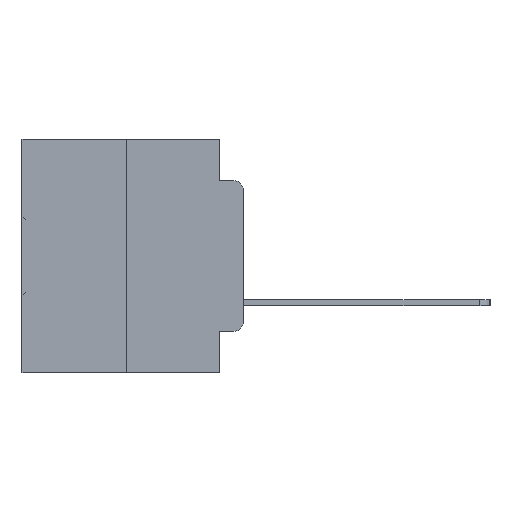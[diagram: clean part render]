
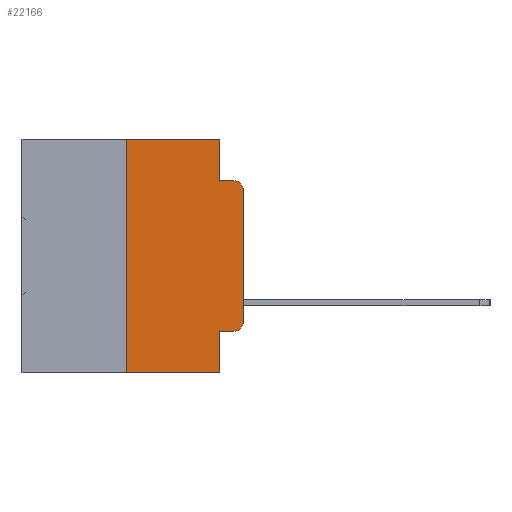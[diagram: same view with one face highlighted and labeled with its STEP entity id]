
A CAD part, left-side view. The second image highlights one B-rep face of the part: STEP entity #22166.
In plain terms, the highlighted planar face has unit normal (-1, 0, 0).
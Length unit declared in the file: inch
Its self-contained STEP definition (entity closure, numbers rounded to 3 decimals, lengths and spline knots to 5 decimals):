
#109 = DIRECTION ( 'NONE',  ( 0., 0., 1. ) ) ;
#383 = CARTESIAN_POINT ( 'NONE',  ( 0., 0.473, -0.5 ) ) ;
#1084 = CARTESIAN_POINT ( 'NONE',  ( 0., 0.051, -0.4115 ) ) ;
#1219 = VERTEX_POINT ( 'NONE', #2418 ) ;
#1689 = AXIS2_PLACEMENT_3D ( 'NONE', #15509, #33247, #18102 ) ;
#1875 = ORIENTED_EDGE ( 'NONE', *, *, #22850, .F. ) ;
#2098 = LINE ( 'NONE', #383, #22154 ) ;
#2418 = CARTESIAN_POINT ( 'NONE',  ( 0., 0.25, -0.5 ) ) ;
#2721 = ORIENTED_EDGE ( 'NONE', *, *, #19456, .F. ) ;
#2844 = VECTOR ( 'NONE', #31445, 39.37008 ) ;
#3057 = VECTOR ( 'NONE', #15112, 39.37008 ) ;
#3071 = CARTESIAN_POINT ( 'NONE',  ( 0., 0.051, -0.0885 ) ) ;
#3792 = CARTESIAN_POINT ( 'NONE',  ( 0., 0.051, 0. ) ) ;
#3800 = CARTESIAN_POINT ( 'NONE',  ( 0., 0.02, -0.4115 ) ) ;
#4260 = DIRECTION ( 'NONE',  ( -1., 0., 0. ) ) ;
#4537 = LINE ( 'NONE', #3071, #2844 ) ;
#5016 = FACE_OUTER_BOUND ( 'NONE', #20043, .T. ) ;
#5463 = EDGE_CURVE ( 'NONE', #11853, #7106, #16193, .T. ) ;
#6418 = LINE ( 'NONE', #9921, #3057 ) ;
#6917 = ORIENTED_EDGE ( 'NONE', *, *, #26914, .T. ) ;
#6985 = CARTESIAN_POINT ( 'NONE',  ( 0., 0.051, 0. ) ) ;
#7106 = VERTEX_POINT ( 'NONE', #3800 ) ;
#7286 = EDGE_CURVE ( 'NONE', #7495, #8517, #6418, .T. ) ;
#7331 = CIRCLE ( 'NONE', #1689, 0.02 ) ;
#7495 = VERTEX_POINT ( 'NONE', #10803 ) ;
#7937 = CARTESIAN_POINT ( 'NONE',  ( 0., 0.473, 0. ) ) ;
#8517 = VERTEX_POINT ( 'NONE', #6985 ) ;
#9064 = EDGE_CURVE ( 'NONE', #11853, #24849, #19349, .T. ) ;
#9236 = DIRECTION ( 'NONE',  ( 0., -1., 0. ) ) ;
#9921 = CARTESIAN_POINT ( 'NONE',  ( 0., 0.473, 0. ) ) ;
#10445 = VECTOR ( 'NONE', #28648, 39.37008 ) ;
#10682 = ORIENTED_EDGE ( 'NONE', *, *, #14294, .F. ) ;
#10803 = CARTESIAN_POINT ( 'NONE',  ( 0., 0.25, 0. ) ) ;
#11853 = VERTEX_POINT ( 'NONE', #23252 ) ;
#12531 = CARTESIAN_POINT ( 'NONE',  ( 0., 0.051, 0. ) ) ;
#13081 = VECTOR ( 'NONE', #15116, 39.37008 ) ;
#13398 = CARTESIAN_POINT ( 'NONE',  ( 0., 0.25, 0. ) ) ;
#13897 = LINE ( 'NONE', #12531, #13081 ) ;
#14112 = VERTEX_POINT ( 'NONE', #32960 ) ;
#14294 = EDGE_CURVE ( 'NONE', #1219, #7495, #27599, .T. ) ;
#14650 = CARTESIAN_POINT ( 'NONE',  ( 0., 0.051, -0.0885 ) ) ;
#15112 = DIRECTION ( 'NONE',  ( 0., -1., 0. ) ) ;
#15116 = DIRECTION ( 'NONE',  ( 0., 0., -1. ) ) ;
#15509 = CARTESIAN_POINT ( 'NONE',  ( 0., 0.02, -0.3915 ) ) ;
#15815 = DIRECTION ( 'NONE',  ( 1., 0., 0. ) ) ;
#16193 = LINE ( 'NONE', #1084, #22183 ) ;
#16438 = AXIS2_PLACEMENT_3D ( 'NONE', #7937, #15815, #33530 ) ;
#18102 = DIRECTION ( 'NONE',  ( 0., 0., -1. ) ) ;
#19349 = LINE ( 'NONE', #3792, #32027 ) ;
#19456 = EDGE_CURVE ( 'NONE', #8517, #25572, #13897, .T. ) ;
#19931 = CARTESIAN_POINT ( 'NONE',  ( 0., 0.02, -0.1085 ) ) ;
#20043 = EDGE_LOOP ( 'NONE', ( #27113, #21157, #1875, #2721, #30262, #10682, #31060, #31845, #32626, #6917 ) ) ;
#20969 = EDGE_CURVE ( 'NONE', #1219, #24849, #2098, .T. ) ;
#21157 = ORIENTED_EDGE ( 'NONE', *, *, #31353, .T. ) ;
#22154 = VECTOR ( 'NONE', #23950, 39.37008 ) ;
#22166 = ADVANCED_FACE ( 'NONE', ( #5016 ), #28498, .F. ) ;
#22183 = VECTOR ( 'NONE', #9236, 39.37008 ) ;
#22481 = DIRECTION ( 'NONE',  ( 0., 0., -1. ) ) ;
#22850 = EDGE_CURVE ( 'NONE', #25572, #27239, #4537, .T. ) ;
#23066 = CIRCLE ( 'NONE', #29163, 0.02 ) ;
#23252 = CARTESIAN_POINT ( 'NONE',  ( 0., 0.051, -0.4115 ) ) ;
#23852 = CARTESIAN_POINT ( 'NONE',  ( 0., 0.051, -0.5 ) ) ;
#23950 = DIRECTION ( 'NONE',  ( 0., -1., 0. ) ) ;
#24071 = LINE ( 'NONE', #26122, #10445 ) ;
#24426 = CARTESIAN_POINT ( 'NONE',  ( 0., 0.02, -0.0885 ) ) ;
#24849 = VERTEX_POINT ( 'NONE', #23852 ) ;
#25572 = VERTEX_POINT ( 'NONE', #14650 ) ;
#26015 = VECTOR ( 'NONE', #109, 39.37008 ) ;
#26122 = CARTESIAN_POINT ( 'NONE',  ( 0., 0., 0. ) ) ;
#26914 = EDGE_CURVE ( 'NONE', #7106, #14112, #7331, .T. ) ;
#27113 = ORIENTED_EDGE ( 'NONE', *, *, #33012, .T. ) ;
#27239 = VERTEX_POINT ( 'NONE', #24426 ) ;
#27599 = LINE ( 'NONE', #13398, #26015 ) ;
#28498 = PLANE ( 'NONE',  #16438 ) ;
#28648 = DIRECTION ( 'NONE',  ( 0., 0., 1. ) ) ;
#28743 = CARTESIAN_POINT ( 'NONE',  ( 0., 0., -0.1085 ) ) ;
#29163 = AXIS2_PLACEMENT_3D ( 'NONE', #19931, #4260, #22481 ) ;
#30262 = ORIENTED_EDGE ( 'NONE', *, *, #7286, .F. ) ;
#30402 = VERTEX_POINT ( 'NONE', #28743 ) ;
#31060 = ORIENTED_EDGE ( 'NONE', *, *, #20969, .T. ) ;
#31353 = EDGE_CURVE ( 'NONE', #30402, #27239, #23066, .T. ) ;
#31445 = DIRECTION ( 'NONE',  ( 0., -1., 0. ) ) ;
#31845 = ORIENTED_EDGE ( 'NONE', *, *, #9064, .F. ) ;
#32027 = VECTOR ( 'NONE', #32227, 39.37008 ) ;
#32227 = DIRECTION ( 'NONE',  ( 0., 0., -1. ) ) ;
#32626 = ORIENTED_EDGE ( 'NONE', *, *, #5463, .T. ) ;
#32960 = CARTESIAN_POINT ( 'NONE',  ( 0., 0., -0.3915 ) ) ;
#33012 = EDGE_CURVE ( 'NONE', #14112, #30402, #24071, .T. ) ;
#33247 = DIRECTION ( 'NONE',  ( -1., 0., 0. ) ) ;
#33530 = DIRECTION ( 'NONE',  ( 0., 0., -1. ) ) ;
